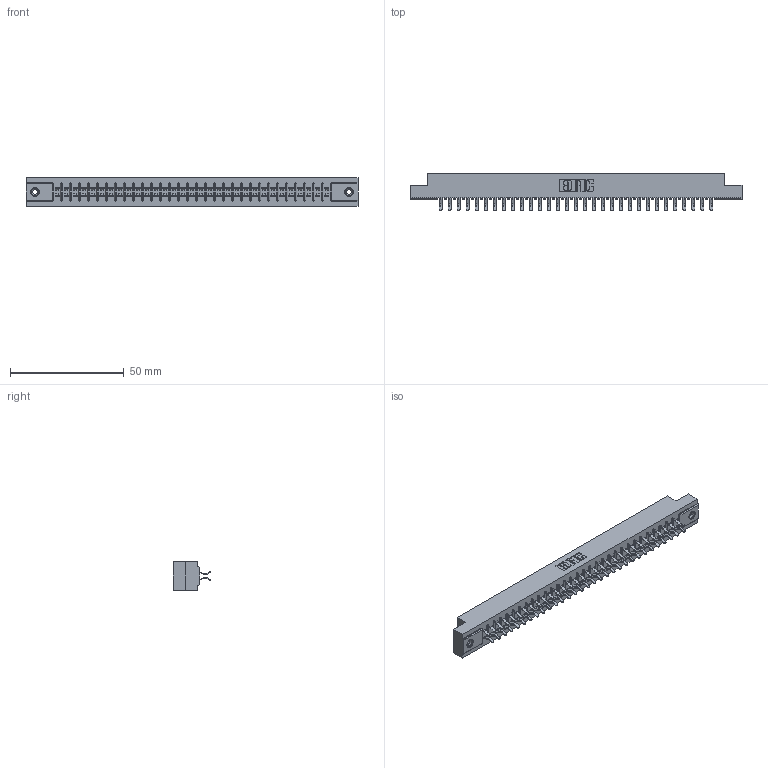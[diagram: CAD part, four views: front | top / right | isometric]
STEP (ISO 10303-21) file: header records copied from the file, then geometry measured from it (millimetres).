
FILE_DESCRIPTION (( 'STEP AP203' ), '1' );
FILE_NAME ('305-062-556-508.STEP', '2019-09-10T02:20:59', ( '' ), ( '' ), 'SwSTEP 2.0', 'SolidWorks 2016', '' );
FILE_SCHEMA (( 'CONFIG_CONTROL_DESIGN' ));
Length unit declared in the file: inch
Products named in the file (4): 345-250-001_345-250-003-102; 305-290-001_556; 305 Part_.156 Dia; 305-062-556-508
Assembly tree (65 placements, depth 2):
  305-062-556-508
    305 Part_.156 Dia
    305-290-001_556  x62
    345-250-001_345-250-003-102  x2
Bounding box: 145.85 x 16.64 x 12.7 mm (x, y, z)
Volume: 14703.9 mm3; surface area: 19184.7 mm2
Topology: 65 solids, 65 shells, 3648 faces, 10465 edges, 6802 vertices
Faces by surface type: plane 2022, cylinder 1486, sphere 124, cone 12, torus 4
Entity records: 36311 total; most frequent: CARTESIAN_POINT 5994, ORIENTED_EDGE 5942, DIRECTION 5821, EDGE_CURVE 2971, LINE 2383, VECTOR 2383, VERTEX_POINT 1892, AXIS2_PLACEMENT_3D 1719
